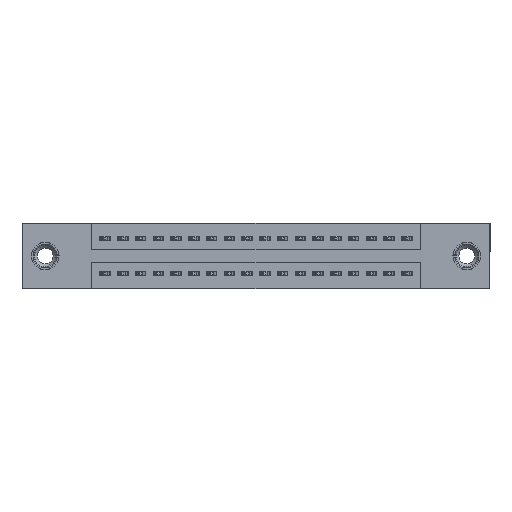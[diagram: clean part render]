
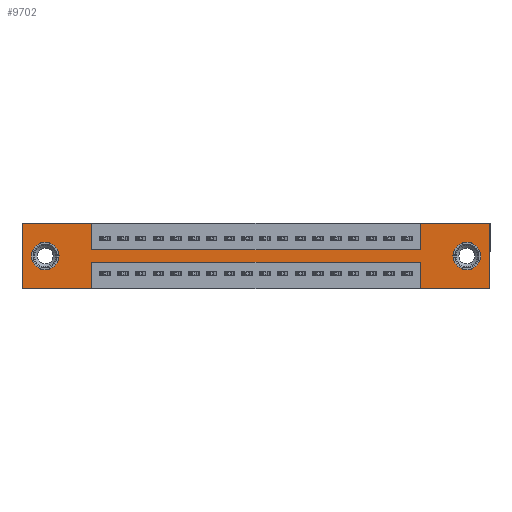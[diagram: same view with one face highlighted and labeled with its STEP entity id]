
A CAD part, front view. The second image highlights one B-rep face of the part: STEP entity #9702.
In plain terms, the highlighted planar face has unit normal (0, -1, 0).
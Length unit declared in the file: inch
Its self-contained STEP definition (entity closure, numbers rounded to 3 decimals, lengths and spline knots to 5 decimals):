
#116 = DIRECTION ( 'NONE',  ( -1., 0., 0. ) ) ;
#184 = DIRECTION ( 'NONE',  ( 0., 0., -1. ) ) ;
#321 = LINE ( 'NONE', #16684, #11844 ) ;
#923 = VERTEX_POINT ( 'NONE', #5670 ) ;
#962 = CARTESIAN_POINT ( 'NONE',  ( 0., 0., 0. ) ) ;
#1042 = VECTOR ( 'NONE', #2658, 39.37008 ) ;
#1558 = ORIENTED_EDGE ( 'NONE', *, *, #18721, .F. ) ;
#1586 = ORIENTED_EDGE ( 'NONE', *, *, #14432, .F. ) ;
#1735 = CARTESIAN_POINT ( 'NONE',  ( 0.3925, 0., 0. ) ) ;
#2080 = AXIS2_PLACEMENT_3D ( 'NONE', #18238, #9188, #184 ) ;
#2222 = CARTESIAN_POINT ( 'NONE',  ( 0.13, 0., -0.185 ) ) ;
#2233 = LINE ( 'NONE', #5543, #8804 ) ;
#2328 = ORIENTED_EDGE ( 'NONE', *, *, #18192, .F. ) ;
#2350 = DIRECTION ( 'NONE',  ( -1., 0., 0. ) ) ;
#2491 = CIRCLE ( 'NONE', #2080, 0.078 ) ;
#2537 = AXIS2_PLACEMENT_3D ( 'NONE', #8718, #17821, #8778 ) ;
#2658 = DIRECTION ( 'NONE',  ( 0., 0., 1. ) ) ;
#2861 = DIRECTION ( 'NONE',  ( 0., 0., 1. ) ) ;
#2872 = LINE ( 'NONE', #10641, #10848 ) ;
#2990 = EDGE_CURVE ( 'NONE', #16479, #5553, #9212, .T. ) ;
#3544 = CARTESIAN_POINT ( 'NONE',  ( 0.13, 0., -0.185 ) ) ;
#3758 = DIRECTION ( 'NONE',  ( 0., 0., 1. ) ) ;
#3872 = LINE ( 'NONE', #6615, #19432 ) ;
#4066 = CARTESIAN_POINT ( 'NONE',  ( 2.2425, 0., -0.22 ) ) ;
#4201 = LINE ( 'NONE', #14996, #15284 ) ;
#4282 = ORIENTED_EDGE ( 'NONE', *, *, #2990, .F. ) ;
#4312 = AXIS2_PLACEMENT_3D ( 'NONE', #2222, #12750, #3758 ) ;
#4380 = CARTESIAN_POINT ( 'NONE',  ( 0.13, 0., -0.107 ) ) ;
#4712 = VERTEX_POINT ( 'NONE', #7842 ) ;
#5061 = DIRECTION ( 'NONE',  ( 0., 0., 1. ) ) ;
#5073 = LINE ( 'NONE', #11644, #1042 ) ;
#5299 = VERTEX_POINT ( 'NONE', #1735 ) ;
#5543 = CARTESIAN_POINT ( 'NONE',  ( 0.3925, 0., 0. ) ) ;
#5553 = VERTEX_POINT ( 'NONE', #13750 ) ;
#5670 = CARTESIAN_POINT ( 'NONE',  ( 2.635, 0., 0. ) ) ;
#5724 = VECTOR ( 'NONE', #14330, 39.37008 ) ;
#5747 = ORIENTED_EDGE ( 'NONE', *, *, #13356, .F. ) ;
#5929 = ORIENTED_EDGE ( 'NONE', *, *, #9508, .F. ) ;
#6415 = AXIS2_PLACEMENT_3D ( 'NONE', #6527, #17088, #8031 ) ;
#6428 = CARTESIAN_POINT ( 'NONE',  ( 0., 0., 0. ) ) ;
#6527 = CARTESIAN_POINT ( 'NONE',  ( 2.505, 0., -0.185 ) ) ;
#6610 = CIRCLE ( 'NONE', #4312, 0.078 ) ;
#6614 = ORIENTED_EDGE ( 'NONE', *, *, #13096, .F. ) ;
#6615 = CARTESIAN_POINT ( 'NONE',  ( 0., 0., 0. ) ) ;
#7425 = DIRECTION ( 'NONE',  ( 1., 0., 0. ) ) ;
#7481 = VERTEX_POINT ( 'NONE', #10557 ) ;
#7842 = CARTESIAN_POINT ( 'NONE',  ( 2.2425, 0., -0.37 ) ) ;
#7945 = CARTESIAN_POINT ( 'NONE',  ( 2.635, 0., 0. ) ) ;
#8031 = DIRECTION ( 'NONE',  ( 0., 0., -1. ) ) ;
#8045 = VERTEX_POINT ( 'NONE', #9085 ) ;
#8254 = ORIENTED_EDGE ( 'NONE', *, *, #12828, .T. ) ;
#8265 = EDGE_CURVE ( 'NONE', #13823, #13037, #10108, .T. ) ;
#8445 = VERTEX_POINT ( 'NONE', #11506 ) ;
#8523 = EDGE_CURVE ( 'NONE', #4712, #16479, #13906, .T. ) ;
#8630 = FACE_BOUND ( 'NONE', #11256, .T. ) ;
#8718 = CARTESIAN_POINT ( 'NONE',  ( 0., 0., -0.37 ) ) ;
#8778 = DIRECTION ( 'NONE',  ( 0., 0., -1. ) ) ;
#8804 = VECTOR ( 'NONE', #16083, 39.37008 ) ;
#8876 = ORIENTED_EDGE ( 'NONE', *, *, #16665, .F. ) ;
#8877 = VECTOR ( 'NONE', #2350, 39.37008 ) ;
#9036 = VERTEX_POINT ( 'NONE', #4380 ) ;
#9085 = CARTESIAN_POINT ( 'NONE',  ( 2.2425, 0., -0.15 ) ) ;
#9188 = DIRECTION ( 'NONE',  ( 0., 1., 0. ) ) ;
#9212 = LINE ( 'NONE', #17283, #5724 ) ;
#9248 = CARTESIAN_POINT ( 'NONE',  ( 0., 0., -0.37 ) ) ;
#9269 = CARTESIAN_POINT ( 'NONE',  ( 2.2425, 0., 0. ) ) ;
#9328 = EDGE_CURVE ( 'NONE', #12137, #17242, #11234, .T. ) ;
#9493 = VERTEX_POINT ( 'NONE', #18834 ) ;
#9508 = EDGE_CURVE ( 'NONE', #8445, #12137, #11934, .T. ) ;
#9702 = ADVANCED_FACE ( 'NONE', ( #13134, #8630, #16686 ), #14830, .T. ) ;
#9738 = CIRCLE ( 'NONE', #13714, 0.078 ) ;
#10108 = CIRCLE ( 'NONE', #6415, 0.078 ) ;
#10330 = ORIENTED_EDGE ( 'NONE', *, *, #9328, .F. ) ;
#10557 = CARTESIAN_POINT ( 'NONE',  ( 0.13, 0., -0.263 ) ) ;
#10641 = CARTESIAN_POINT ( 'NONE',  ( 0., 0., -0.37 ) ) ;
#10848 = VECTOR ( 'NONE', #116, 39.37008 ) ;
#11035 = EDGE_LOOP ( 'NONE', ( #15486, #16739 ) ) ;
#11234 = LINE ( 'NONE', #6428, #15306 ) ;
#11256 = EDGE_LOOP ( 'NONE', ( #8254, #17735 ) ) ;
#11344 = CARTESIAN_POINT ( 'NONE',  ( 0., 0., -0.37 ) ) ;
#11432 = LINE ( 'NONE', #7945, #15038 ) ;
#11506 = CARTESIAN_POINT ( 'NONE',  ( 0.3925, 0., -0.37 ) ) ;
#11644 = CARTESIAN_POINT ( 'NONE',  ( 2.2425, 0., 0. ) ) ;
#11844 = VECTOR ( 'NONE', #13778, 39.37008 ) ;
#11934 = LINE ( 'NONE', #11344, #8877 ) ;
#12077 = EDGE_CURVE ( 'NONE', #13037, #13823, #2491, .T. ) ;
#12137 = VERTEX_POINT ( 'NONE', #9248 ) ;
#12461 = EDGE_LOOP ( 'NONE', ( #5747, #4282, #18272, #19285, #13543, #1586, #6614, #8876, #2328, #1558, #10330, #5929 ) ) ;
#12750 = DIRECTION ( 'NONE',  ( 0., 1., 0. ) ) ;
#12828 = EDGE_CURVE ( 'NONE', #9036, #7481, #9738, .T. ) ;
#13037 = VERTEX_POINT ( 'NONE', #17526 ) ;
#13096 = EDGE_CURVE ( 'NONE', #8045, #16819, #5073, .T. ) ;
#13134 = FACE_BOUND ( 'NONE', #11035, .T. ) ;
#13156 = CARTESIAN_POINT ( 'NONE',  ( 2.505, 0., -0.107 ) ) ;
#13356 = EDGE_CURVE ( 'NONE', #5553, #8445, #321, .T. ) ;
#13377 = CARTESIAN_POINT ( 'NONE',  ( 2.2425, 0., -0.37 ) ) ;
#13543 = ORIENTED_EDGE ( 'NONE', *, *, #16904, .F. ) ;
#13714 = AXIS2_PLACEMENT_3D ( 'NONE', #3544, #14066, #5061 ) ;
#13750 = CARTESIAN_POINT ( 'NONE',  ( 0.3925, 0., -0.22 ) ) ;
#13778 = DIRECTION ( 'NONE',  ( 0., 0., -1. ) ) ;
#13823 = VERTEX_POINT ( 'NONE', #13156 ) ;
#13841 = VERTEX_POINT ( 'NONE', #19241 ) ;
#13906 = LINE ( 'NONE', #13377, #17900 ) ;
#14066 = DIRECTION ( 'NONE',  ( 0., 1., 0. ) ) ;
#14330 = DIRECTION ( 'NONE',  ( -1., 0., 0. ) ) ;
#14432 = EDGE_CURVE ( 'NONE', #16819, #923, #17026, .T. ) ;
#14830 = PLANE ( 'NONE',  #2537 ) ;
#14996 = CARTESIAN_POINT ( 'NONE',  ( 0.3925, 0., -0.15 ) ) ;
#15038 = VECTOR ( 'NONE', #17014, 39.37008 ) ;
#15284 = VECTOR ( 'NONE', #7425, 39.37008 ) ;
#15306 = VECTOR ( 'NONE', #18506, 39.37008 ) ;
#15446 = EDGE_CURVE ( 'NONE', #13841, #4712, #2872, .T. ) ;
#15486 = ORIENTED_EDGE ( 'NONE', *, *, #8265, .T. ) ;
#15702 = EDGE_CURVE ( 'NONE', #7481, #9036, #6610, .T. ) ;
#15999 = DIRECTION ( 'NONE',  ( 1., 0., 0. ) ) ;
#16083 = DIRECTION ( 'NONE',  ( 0., 0., -1. ) ) ;
#16479 = VERTEX_POINT ( 'NONE', #4066 ) ;
#16665 = EDGE_CURVE ( 'NONE', #9493, #8045, #4201, .T. ) ;
#16684 = CARTESIAN_POINT ( 'NONE',  ( 0.3925, 0., -0.37 ) ) ;
#16686 = FACE_OUTER_BOUND ( 'NONE', #12461, .T. ) ;
#16739 = ORIENTED_EDGE ( 'NONE', *, *, #12077, .T. ) ;
#16819 = VERTEX_POINT ( 'NONE', #9269 ) ;
#16904 = EDGE_CURVE ( 'NONE', #923, #13841, #11432, .T. ) ;
#17014 = DIRECTION ( 'NONE',  ( 0., 0., -1. ) ) ;
#17026 = LINE ( 'NONE', #962, #18442 ) ;
#17088 = DIRECTION ( 'NONE',  ( 0., 1., 0. ) ) ;
#17180 = DIRECTION ( 'NONE',  ( 1., 0., 0. ) ) ;
#17242 = VERTEX_POINT ( 'NONE', #17767 ) ;
#17283 = CARTESIAN_POINT ( 'NONE',  ( 0.3925, 0., -0.22 ) ) ;
#17526 = CARTESIAN_POINT ( 'NONE',  ( 2.505, 0., -0.263 ) ) ;
#17735 = ORIENTED_EDGE ( 'NONE', *, *, #15702, .T. ) ;
#17767 = CARTESIAN_POINT ( 'NONE',  ( 0., 0., 0. ) ) ;
#17821 = DIRECTION ( 'NONE',  ( 0., -1., 0. ) ) ;
#17900 = VECTOR ( 'NONE', #2861, 39.37008 ) ;
#18192 = EDGE_CURVE ( 'NONE', #5299, #9493, #2233, .T. ) ;
#18238 = CARTESIAN_POINT ( 'NONE',  ( 2.505, 0., -0.185 ) ) ;
#18272 = ORIENTED_EDGE ( 'NONE', *, *, #8523, .F. ) ;
#18442 = VECTOR ( 'NONE', #15999, 39.37008 ) ;
#18506 = DIRECTION ( 'NONE',  ( 0., 0., 1. ) ) ;
#18721 = EDGE_CURVE ( 'NONE', #17242, #5299, #3872, .T. ) ;
#18834 = CARTESIAN_POINT ( 'NONE',  ( 0.3925, 0., -0.15 ) ) ;
#19241 = CARTESIAN_POINT ( 'NONE',  ( 2.635, 0., -0.37 ) ) ;
#19285 = ORIENTED_EDGE ( 'NONE', *, *, #15446, .F. ) ;
#19432 = VECTOR ( 'NONE', #17180, 39.37008 ) ;
